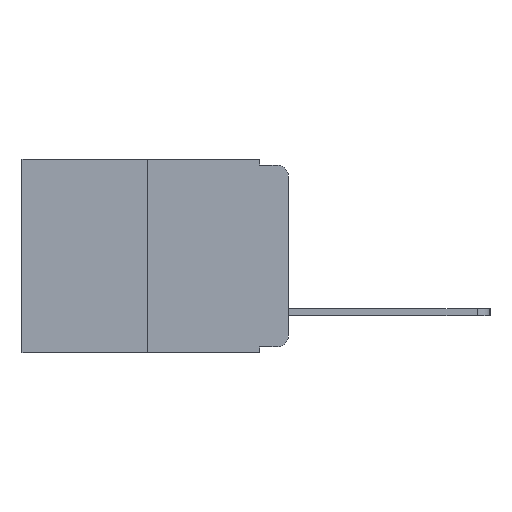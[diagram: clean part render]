
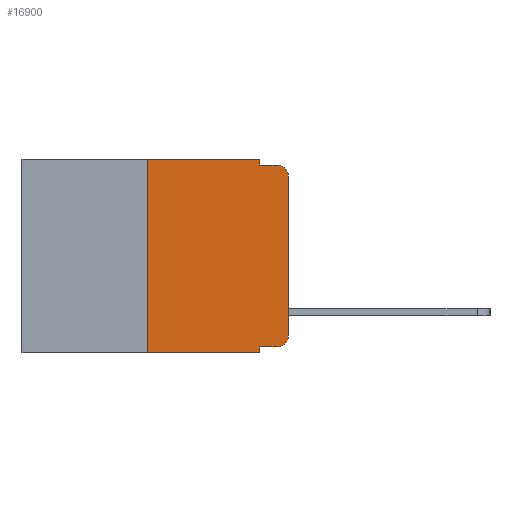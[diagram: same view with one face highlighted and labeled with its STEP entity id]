
A CAD part, left-side view. The second image highlights one B-rep face of the part: STEP entity #16900.
In plain terms, the highlighted planar face has unit normal (-1, 0, 0).
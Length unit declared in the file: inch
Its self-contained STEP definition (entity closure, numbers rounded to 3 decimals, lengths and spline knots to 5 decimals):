
#126 = VECTOR ( 'NONE', #5033, 39.37008 ) ;
#130 = DIRECTION ( 'NONE',  ( 0., 0., -1. ) ) ;
#549 = VERTEX_POINT ( 'NONE', #15264 ) ;
#608 = ORIENTED_EDGE ( 'NONE', *, *, #15553, .T. ) ;
#639 = DIRECTION ( 'NONE',  ( 0., -1., 0. ) ) ;
#685 = LINE ( 'NONE', #3458, #126 ) ;
#970 = EDGE_CURVE ( 'NONE', #16372, #17652, #6215, .T. ) ;
#1011 = LINE ( 'NONE', #18880, #16356 ) ;
#1409 = VECTOR ( 'NONE', #15902, 39.37008 ) ;
#1562 = CARTESIAN_POINT ( 'NONE',  ( 0., 0., 0. ) ) ;
#1898 = LINE ( 'NONE', #14343, #1409 ) ;
#2695 = VECTOR ( 'NONE', #17214, 39.37008 ) ;
#2955 = EDGE_LOOP ( 'NONE', ( #608, #9582, #10097, #18399, #10599, #11104, #15256, #19329, #3646, #7825 ) ) ;
#3458 = CARTESIAN_POINT ( 'NONE',  ( 0., 0.051, 0. ) ) ;
#3560 = FACE_OUTER_BOUND ( 'NONE', #2955, .T. ) ;
#3646 = ORIENTED_EDGE ( 'NONE', *, *, #9214, .T. ) ;
#3774 = CARTESIAN_POINT ( 'NONE',  ( 0., 0.02, -0.313 ) ) ;
#4181 = DIRECTION ( 'NONE',  ( 1., 0., 0. ) ) ;
#4438 = CARTESIAN_POINT ( 'NONE',  ( 0., 0., -0.03 ) ) ;
#4646 = VERTEX_POINT ( 'NONE', #7457 ) ;
#4692 = CARTESIAN_POINT ( 'NONE',  ( 0., 0.02, -0.333 ) ) ;
#4979 = DIRECTION ( 'NONE',  ( 0., -1., 0. ) ) ;
#5033 = DIRECTION ( 'NONE',  ( 0., 0., -1. ) ) ;
#5187 = VERTEX_POINT ( 'NONE', #4692 ) ;
#5370 = DIRECTION ( 'NONE',  ( 0., 0., -1. ) ) ;
#5672 = CARTESIAN_POINT ( 'NONE',  ( 0., 0.473, -0.343 ) ) ;
#5989 = CARTESIAN_POINT ( 'NONE',  ( 0., 0.051, 0. ) ) ;
#6205 = AXIS2_PLACEMENT_3D ( 'NONE', #13661, #4181, #15225 ) ;
#6215 = LINE ( 'NONE', #5672, #9943 ) ;
#6885 = LINE ( 'NONE', #20156, #2695 ) ;
#7457 = CARTESIAN_POINT ( 'NONE',  ( 0., 0.051, -0.333 ) ) ;
#7567 = DIRECTION ( 'NONE',  ( 0., 0., -1. ) ) ;
#7825 = ORIENTED_EDGE ( 'NONE', *, *, #8127, .T. ) ;
#8127 = EDGE_CURVE ( 'NONE', #5187, #10738, #20166, .T. ) ;
#8580 = CARTESIAN_POINT ( 'NONE',  ( 0., 0.051, -0.01 ) ) ;
#9116 = CARTESIAN_POINT ( 'NONE',  ( 0., 0.25, -0.343 ) ) ;
#9214 = EDGE_CURVE ( 'NONE', #4646, #5187, #1011, .T. ) ;
#9329 = VECTOR ( 'NONE', #15803, 39.37008 ) ;
#9582 = ORIENTED_EDGE ( 'NONE', *, *, #14499, .T. ) ;
#9618 = CIRCLE ( 'NONE', #17911, 0.02 ) ;
#9712 = DIRECTION ( 'NONE',  ( -1., 0., 0. ) ) ;
#9943 = VECTOR ( 'NONE', #4979, 39.37008 ) ;
#10097 = ORIENTED_EDGE ( 'NONE', *, *, #13464, .F. ) ;
#10292 = EDGE_CURVE ( 'NONE', #4646, #17652, #685, .T. ) ;
#10549 = LINE ( 'NONE', #8580, #17896 ) ;
#10599 = ORIENTED_EDGE ( 'NONE', *, *, #14386, .F. ) ;
#10738 = VERTEX_POINT ( 'NONE', #12455 ) ;
#10861 = VECTOR ( 'NONE', #7567, 39.37008 ) ;
#10955 = CARTESIAN_POINT ( 'NONE',  ( 0., 0.051, -0.01 ) ) ;
#11104 = ORIENTED_EDGE ( 'NONE', *, *, #11365, .F. ) ;
#11365 = EDGE_CURVE ( 'NONE', #16372, #549, #1898, .T. ) ;
#12421 = EDGE_CURVE ( 'NONE', #12423, #13778, #14745, .T. ) ;
#12423 = VERTEX_POINT ( 'NONE', #5989 ) ;
#12455 = CARTESIAN_POINT ( 'NONE',  ( 0., 0., -0.313 ) ) ;
#12478 = AXIS2_PLACEMENT_3D ( 'NONE', #3774, #14842, #5370 ) ;
#13464 = EDGE_CURVE ( 'NONE', #13778, #13822, #10549, .T. ) ;
#13538 = LINE ( 'NONE', #1562, #9329 ) ;
#13661 = CARTESIAN_POINT ( 'NONE',  ( 0., 0.473, 0. ) ) ;
#13778 = VERTEX_POINT ( 'NONE', #10955 ) ;
#13822 = VERTEX_POINT ( 'NONE', #20307 ) ;
#14243 = DIRECTION ( 'NONE',  ( 0., -1., 0. ) ) ;
#14343 = CARTESIAN_POINT ( 'NONE',  ( 0., 0.25, 0. ) ) ;
#14386 = EDGE_CURVE ( 'NONE', #549, #12423, #6885, .T. ) ;
#14499 = EDGE_CURVE ( 'NONE', #17023, #13822, #9618, .T. ) ;
#14745 = LINE ( 'NONE', #17029, #10861 ) ;
#14842 = DIRECTION ( 'NONE',  ( -1., 0., 0. ) ) ;
#15225 = DIRECTION ( 'NONE',  ( 0., 0., -1. ) ) ;
#15256 = ORIENTED_EDGE ( 'NONE', *, *, #970, .T. ) ;
#15264 = CARTESIAN_POINT ( 'NONE',  ( 0., 0.25, 0. ) ) ;
#15553 = EDGE_CURVE ( 'NONE', #10738, #17023, #13538, .T. ) ;
#15803 = DIRECTION ( 'NONE',  ( 0., 0., 1. ) ) ;
#15902 = DIRECTION ( 'NONE',  ( 0., 0., 1. ) ) ;
#16356 = VECTOR ( 'NONE', #14243, 39.37008 ) ;
#16372 = VERTEX_POINT ( 'NONE', #9116 ) ;
#16900 = ADVANCED_FACE ( 'NONE', ( #3560 ), #18276, .F. ) ;
#17023 = VERTEX_POINT ( 'NONE', #4438 ) ;
#17029 = CARTESIAN_POINT ( 'NONE',  ( 0., 0.051, 0. ) ) ;
#17214 = DIRECTION ( 'NONE',  ( 0., -1., 0. ) ) ;
#17652 = VERTEX_POINT ( 'NONE', #18595 ) ;
#17896 = VECTOR ( 'NONE', #639, 39.37008 ) ;
#17911 = AXIS2_PLACEMENT_3D ( 'NONE', #19042, #9712, #130 ) ;
#18276 = PLANE ( 'NONE',  #6205 ) ;
#18399 = ORIENTED_EDGE ( 'NONE', *, *, #12421, .F. ) ;
#18595 = CARTESIAN_POINT ( 'NONE',  ( 0., 0.051, -0.343 ) ) ;
#18880 = CARTESIAN_POINT ( 'NONE',  ( 0., 0.051, -0.333 ) ) ;
#19042 = CARTESIAN_POINT ( 'NONE',  ( 0., 0.02, -0.03 ) ) ;
#19329 = ORIENTED_EDGE ( 'NONE', *, *, #10292, .F. ) ;
#20156 = CARTESIAN_POINT ( 'NONE',  ( 0., 0.473, 0. ) ) ;
#20166 = CIRCLE ( 'NONE', #12478, 0.02 ) ;
#20307 = CARTESIAN_POINT ( 'NONE',  ( 0., 0.02, -0.01 ) ) ;
